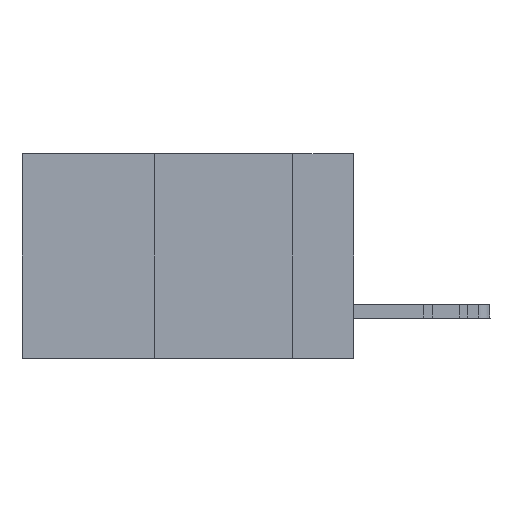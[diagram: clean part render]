
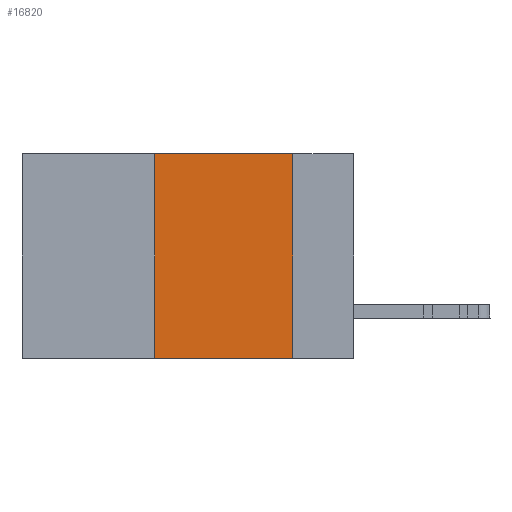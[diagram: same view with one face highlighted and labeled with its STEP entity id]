
A CAD part, left-side view. The second image highlights one B-rep face of the part: STEP entity #16820.
In plain terms, the highlighted planar face has unit normal (-1, 0, 0).
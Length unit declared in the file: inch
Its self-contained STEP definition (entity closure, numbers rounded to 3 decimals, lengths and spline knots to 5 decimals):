
#1511 = PLANE ( 'NONE',  #23615 ) ;
#2384 = VECTOR ( 'NONE', #33196, 39.37008 ) ;
#5514 = CARTESIAN_POINT ( 'NONE',  ( 0., 0.36, -0.37 ) ) ;
#8165 = VECTOR ( 'NONE', #24019, 39.37008 ) ;
#8417 = ORIENTED_EDGE ( 'NONE', *, *, #15115, .F. ) ;
#9236 = VECTOR ( 'NONE', #34049, 39.37008 ) ;
#9520 = ORIENTED_EDGE ( 'NONE', *, *, #43262, .F. ) ;
#9572 = LINE ( 'NONE', #22937, #9236 ) ;
#9761 = CARTESIAN_POINT ( 'NONE',  ( 0., 0.6, -0.37 ) ) ;
#9979 = LINE ( 'NONE', #9761, #8165 ) ;
#10023 = CARTESIAN_POINT ( 'NONE',  ( 0., 0.36, 0. ) ) ;
#10694 = EDGE_CURVE ( 'NONE', #28425, #25802, #9979, .T. ) ;
#12924 = LINE ( 'NONE', #43216, #2384 ) ;
#13151 = DIRECTION ( 'NONE',  ( 0., 0., 1. ) ) ;
#15115 = EDGE_CURVE ( 'NONE', #28425, #40356, #30728, .T. ) ;
#15120 = CARTESIAN_POINT ( 'NONE',  ( 0., 0.6, 0. ) ) ;
#15704 = CARTESIAN_POINT ( 'NONE',  ( 0., 0.11, -0.37 ) ) ;
#16820 = ADVANCED_FACE ( 'NONE', ( #32057 ), #1511, .F. ) ;
#17169 = VERTEX_POINT ( 'NONE', #24680 ) ;
#22937 = CARTESIAN_POINT ( 'NONE',  ( 0., 0.6, 0. ) ) ;
#23615 = AXIS2_PLACEMENT_3D ( 'NONE', #15120, #28713, #24731 ) ;
#24019 = DIRECTION ( 'NONE',  ( 0., -1., 0. ) ) ;
#24680 = CARTESIAN_POINT ( 'NONE',  ( 0., 0.11, 0. ) ) ;
#24731 = DIRECTION ( 'NONE',  ( 0., 0., -1. ) ) ;
#25802 = VERTEX_POINT ( 'NONE', #15704 ) ;
#28197 = ORIENTED_EDGE ( 'NONE', *, *, #35656, .F. ) ;
#28425 = VERTEX_POINT ( 'NONE', #5514 ) ;
#28713 = DIRECTION ( 'NONE',  ( 1., 0., 0. ) ) ;
#30651 = EDGE_LOOP ( 'NONE', ( #9520, #28197, #8417, #43086 ) ) ;
#30728 = LINE ( 'NONE', #10023, #32074 ) ;
#32057 = FACE_OUTER_BOUND ( 'NONE', #30651, .T. ) ;
#32074 = VECTOR ( 'NONE', #13151, 39.37008 ) ;
#33196 = DIRECTION ( 'NONE',  ( 0., 0., -1. ) ) ;
#34049 = DIRECTION ( 'NONE',  ( 0., -1., 0. ) ) ;
#35656 = EDGE_CURVE ( 'NONE', #40356, #17169, #9572, .T. ) ;
#40356 = VERTEX_POINT ( 'NONE', #42271 ) ;
#42271 = CARTESIAN_POINT ( 'NONE',  ( 0., 0.36, 0. ) ) ;
#43086 = ORIENTED_EDGE ( 'NONE', *, *, #10694, .T. ) ;
#43216 = CARTESIAN_POINT ( 'NONE',  ( 0., 0.11, 0. ) ) ;
#43262 = EDGE_CURVE ( 'NONE', #17169, #25802, #12924, .T. ) ;
